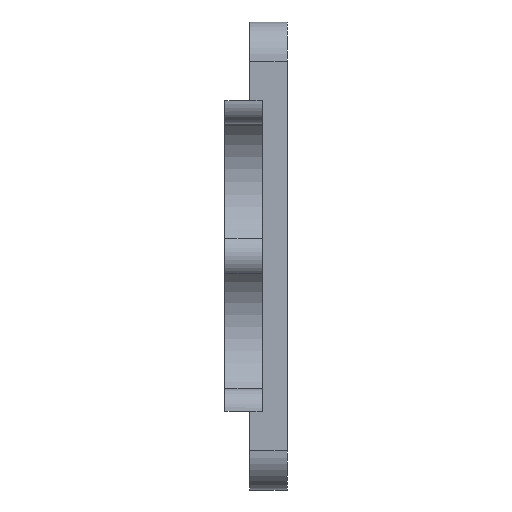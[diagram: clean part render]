
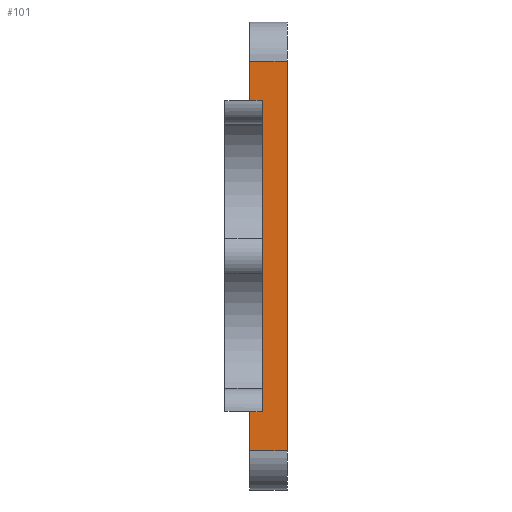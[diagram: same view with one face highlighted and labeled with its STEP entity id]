
A CAD part, left-side view. The second image highlights one B-rep face of the part: STEP entity #101.
In plain terms, the highlighted planar face has unit normal (-1, 0, 0).
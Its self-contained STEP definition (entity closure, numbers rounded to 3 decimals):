
#5 = VERTEX_POINT ( 'NONE', #762 ) ;
#12 = VERTEX_POINT ( 'NONE', #842 ) ;
#13 = CARTESIAN_POINT ( 'NONE',  ( 0., -1.27, 0. ) ) ;
#42 = ORIENTED_EDGE ( 'NONE', *, *, #379, .F. ) ;
#64 = EDGE_CURVE ( 'NONE', #982, #924, #173, .T. ) ;
#70 = EDGE_CURVE ( 'NONE', #12, #764, #502, .T. ) ;
#76 = ORIENTED_EDGE ( 'NONE', *, *, #429, .T. ) ;
#96 = VECTOR ( 'NONE', #140, 1000. ) ;
#101 = ADVANCED_FACE ( 'NONE', ( #1055 ), #639, .F. ) ;
#111 = EDGE_CURVE ( 'NONE', #5, #12, #295, .T. ) ;
#118 = VECTOR ( 'NONE', #1075, 1000. ) ;
#140 = DIRECTION ( 'NONE',  ( 0., 0., -1. ) ) ;
#173 = LINE ( 'NONE', #694, #255 ) ;
#221 = CARTESIAN_POINT ( 'NONE',  ( 0., -1.27, 0. ) ) ;
#253 = VERTEX_POINT ( 'NONE', #1068 ) ;
#255 = VECTOR ( 'NONE', #269, 1000. ) ;
#269 = DIRECTION ( 'NONE',  ( 0., 0., -1. ) ) ;
#272 = EDGE_LOOP ( 'NONE', ( #1038, #550, #76, #42, #532, #1026, #1067, #579 ) ) ;
#273 = LINE ( 'NONE', #759, #784 ) ;
#281 = EDGE_CURVE ( 'NONE', #982, #996, #830, .T. ) ;
#295 = LINE ( 'NONE', #884, #96 ) ;
#305 = VECTOR ( 'NONE', #562, 1000. ) ;
#313 = CARTESIAN_POINT ( 'NONE',  ( 0., -1.905, -19.878 ) ) ;
#329 = EDGE_CURVE ( 'NONE', #604, #924, #447, .T. ) ;
#351 = DIRECTION ( 'NONE',  ( 0., 0., -1. ) ) ;
#379 = EDGE_CURVE ( 'NONE', #5, #253, #273, .T. ) ;
#398 = VECTOR ( 'NONE', #542, 1000. ) ;
#417 = VECTOR ( 'NONE', #351, 1000. ) ;
#424 = CARTESIAN_POINT ( 'NONE',  ( 0., -1.27, -2. ) ) ;
#429 = EDGE_CURVE ( 'NONE', #996, #253, #1034, .T. ) ;
#447 = LINE ( 'NONE', #926, #398 ) ;
#502 = LINE ( 'NONE', #313, #1047 ) ;
#506 = AXIS2_PLACEMENT_3D ( 'NONE', #892, #568, #798 ) ;
#532 = ORIENTED_EDGE ( 'NONE', *, *, #111, .T. ) ;
#542 = DIRECTION ( 'NONE',  ( 0., -1., 0. ) ) ;
#545 = CARTESIAN_POINT ( 'NONE',  ( 0., -3.175, -21.876 ) ) ;
#550 = ORIENTED_EDGE ( 'NONE', *, *, #281, .T. ) ;
#562 = DIRECTION ( 'NONE',  ( 0., 0., -1. ) ) ;
#568 = DIRECTION ( 'NONE',  ( 1., 0., 0. ) ) ;
#579 = ORIENTED_EDGE ( 'NONE', *, *, #329, .T. ) ;
#604 = VERTEX_POINT ( 'NONE', #1053 ) ;
#611 = DIRECTION ( 'NONE',  ( 0., 1., 0. ) ) ;
#614 = CARTESIAN_POINT ( 'NONE',  ( 0., -3.175, -2. ) ) ;
#630 = CARTESIAN_POINT ( 'NONE',  ( 0., -1.27, -2. ) ) ;
#639 = PLANE ( 'NONE',  #506 ) ;
#694 = CARTESIAN_POINT ( 'NONE',  ( 0., -3.175, 0. ) ) ;
#700 = EDGE_CURVE ( 'NONE', #764, #604, #811, .T. ) ;
#757 = CARTESIAN_POINT ( 'NONE',  ( 0., -1.27, -19.878 ) ) ;
#759 = CARTESIAN_POINT ( 'NONE',  ( 0., -1.905, -3.998 ) ) ;
#762 = CARTESIAN_POINT ( 'NONE',  ( 0., -1.905, -3.998 ) ) ;
#764 = VERTEX_POINT ( 'NONE', #757 ) ;
#784 = VECTOR ( 'NONE', #611, 1000. ) ;
#798 = DIRECTION ( 'NONE',  ( 0., 0., -1. ) ) ;
#802 = DIRECTION ( 'NONE',  ( 0., 1., 0. ) ) ;
#811 = LINE ( 'NONE', #221, #305 ) ;
#830 = LINE ( 'NONE', #424, #118 ) ;
#842 = CARTESIAN_POINT ( 'NONE',  ( 0., -1.905, -19.878 ) ) ;
#884 = CARTESIAN_POINT ( 'NONE',  ( 0., -1.905, 0. ) ) ;
#892 = CARTESIAN_POINT ( 'NONE',  ( 0., -3.175, 0. ) ) ;
#924 = VERTEX_POINT ( 'NONE', #545 ) ;
#926 = CARTESIAN_POINT ( 'NONE',  ( 0., -3.175, -21.876 ) ) ;
#982 = VERTEX_POINT ( 'NONE', #614 ) ;
#996 = VERTEX_POINT ( 'NONE', #630 ) ;
#1026 = ORIENTED_EDGE ( 'NONE', *, *, #70, .T. ) ;
#1034 = LINE ( 'NONE', #13, #417 ) ;
#1038 = ORIENTED_EDGE ( 'NONE', *, *, #64, .F. ) ;
#1047 = VECTOR ( 'NONE', #802, 1000. ) ;
#1053 = CARTESIAN_POINT ( 'NONE',  ( 0., -1.27, -21.876 ) ) ;
#1055 = FACE_OUTER_BOUND ( 'NONE', #272, .T. ) ;
#1067 = ORIENTED_EDGE ( 'NONE', *, *, #700, .T. ) ;
#1068 = CARTESIAN_POINT ( 'NONE',  ( 0., -1.27, -3.998 ) ) ;
#1075 = DIRECTION ( 'NONE',  ( 0., 1., 0. ) ) ;
